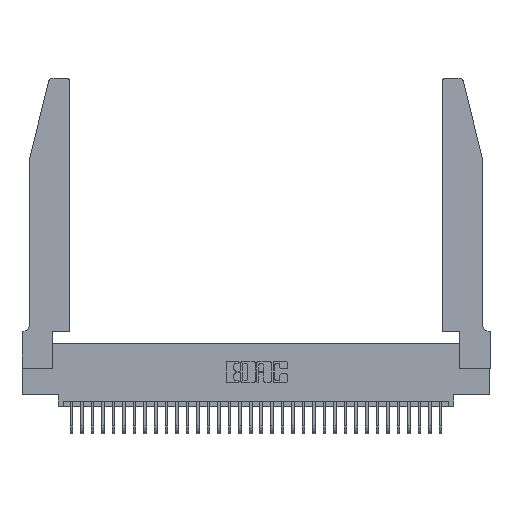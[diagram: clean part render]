
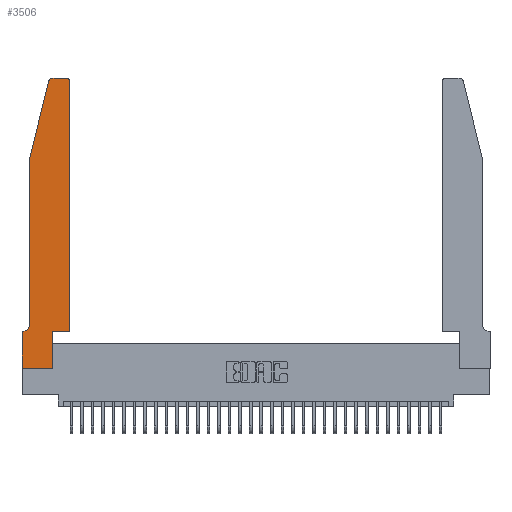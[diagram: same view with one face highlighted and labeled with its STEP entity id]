
A CAD part, top view. The second image highlights one B-rep face of the part: STEP entity #3506.
In plain terms, the highlighted planar face has unit normal (0, 0, 1).
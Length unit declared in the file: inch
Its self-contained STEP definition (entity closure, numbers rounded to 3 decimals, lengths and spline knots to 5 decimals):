
#100 = EDGE_CURVE ( 'NONE', #10285, #5975, #26874, .T. ) ;
#257 = VECTOR ( 'NONE', #12588, 39.37008 ) ;
#809 = AXIS2_PLACEMENT_3D ( 'NONE', #14384, #32097, #16927 ) ;
#1375 = VERTEX_POINT ( 'NONE', #4987 ) ;
#1424 = ORIENTED_EDGE ( 'NONE', *, *, #3995, .T. ) ;
#1667 = LINE ( 'NONE', #10837, #7676 ) ;
#1748 = ORIENTED_EDGE ( 'NONE', *, *, #4830, .T. ) ;
#1762 = DIRECTION ( 'NONE',  ( 0., 0., 1. ) ) ;
#2508 = VERTEX_POINT ( 'NONE', #12590 ) ;
#2565 = VECTOR ( 'NONE', #19138, 39.37008 ) ;
#2974 = EDGE_CURVE ( 'NONE', #5975, #3243, #23541, .T. ) ;
#3184 = CARTESIAN_POINT ( 'NONE',  ( 0.2865, 0.35, 0.37 ) ) ;
#3243 = VERTEX_POINT ( 'NONE', #20461 ) ;
#3506 = ADVANCED_FACE ( 'NONE', ( #21100 ), #26480, .T. ) ;
#3995 = EDGE_CURVE ( 'NONE', #10096, #30530, #20252, .T. ) ;
#4830 = EDGE_CURVE ( 'NONE', #26191, #29279, #29350, .T. ) ;
#4987 = CARTESIAN_POINT ( 'NONE',  ( 0.0055, 0.35, 0.37 ) ) ;
#5156 = CARTESIAN_POINT ( 'NONE',  ( 0., 0., 0.37 ) ) ;
#5867 = VECTOR ( 'NONE', #12984, 39.37008 ) ;
#5939 = VECTOR ( 'NONE', #24804, 39.37008 ) ;
#5963 = VECTOR ( 'NONE', #23634, 39.37008 ) ;
#5975 = VERTEX_POINT ( 'NONE', #12369 ) ;
#6081 = EDGE_CURVE ( 'NONE', #3243, #10096, #18925, .T. ) ;
#7092 = CARTESIAN_POINT ( 'NONE',  ( 0.0755, 2., 0.37 ) ) ;
#7093 = LINE ( 'NONE', #7507, #257 ) ;
#7507 = CARTESIAN_POINT ( 'NONE',  ( 0.4505, 0.35, 0.37 ) ) ;
#7676 = VECTOR ( 'NONE', #25961, 39.37008 ) ;
#7821 = ORIENTED_EDGE ( 'NONE', *, *, #100, .T. ) ;
#7917 = ORIENTED_EDGE ( 'NONE', *, *, #28619, .T. ) ;
#8283 = ORIENTED_EDGE ( 'NONE', *, *, #28003, .T. ) ;
#8808 = CIRCLE ( 'NONE', #809, 0.07 ) ;
#9405 = LINE ( 'NONE', #24055, #2565 ) ;
#9888 = DIRECTION ( 'NONE',  ( 0., -1., 0. ) ) ;
#10096 = VERTEX_POINT ( 'NONE', #30435 ) ;
#10285 = VERTEX_POINT ( 'NONE', #26589 ) ;
#10837 = CARTESIAN_POINT ( 'NONE',  ( 0., 0., 0.37 ) ) ;
#11023 = CARTESIAN_POINT ( 'NONE',  ( 0., 0., 0.37 ) ) ;
#11328 = CARTESIAN_POINT ( 'NONE',  ( 0., 0.35, 0.37 ) ) ;
#11965 = CARTESIAN_POINT ( 'NONE',  ( 0.25487, 2.72718, 0.37 ) ) ;
#12243 = EDGE_CURVE ( 'NONE', #1375, #18558, #29866, .T. ) ;
#12369 = CARTESIAN_POINT ( 'NONE',  ( 0.4505, 2.72, 0.37 ) ) ;
#12539 = EDGE_CURVE ( 'NONE', #30699, #2508, #1667, .T. ) ;
#12588 = DIRECTION ( 'NONE',  ( 1., 0., 0. ) ) ;
#12590 = CARTESIAN_POINT ( 'NONE',  ( 0.2865, 0., 0.37 ) ) ;
#12671 = LINE ( 'NONE', #7092, #5939 ) ;
#12984 = DIRECTION ( 'NONE',  ( 0., 1., 0. ) ) ;
#13039 = DIRECTION ( 'NONE',  ( 0., 0., 1. ) ) ;
#13126 = AXIS2_PLACEMENT_3D ( 'NONE', #11328, #13847, #31569 ) ;
#13847 = DIRECTION ( 'NONE',  ( 0., 0., 1. ) ) ;
#14384 = CARTESIAN_POINT ( 'NONE',  ( 0.0055, 0.42, 0.37 ) ) ;
#15065 = VECTOR ( 'NONE', #9888, 39.37008 ) ;
#15215 = DIRECTION ( 'NONE',  ( -1., 0., 0. ) ) ;
#15487 = EDGE_LOOP ( 'NONE', ( #26988, #1424, #8283, #1748, #27468, #16685, #23437, #31357, #21191, #7917, #7821, #29289 ) ) ;
#16685 = ORIENTED_EDGE ( 'NONE', *, *, #12243, .T. ) ;
#16927 = DIRECTION ( 'NONE',  ( -1., 0., 0. ) ) ;
#16969 = CARTESIAN_POINT ( 'NONE',  ( 0.4205, 2.72, 0.37 ) ) ;
#17240 = DIRECTION ( 'NONE',  ( -1., 0., 0. ) ) ;
#17566 = AXIS2_PLACEMENT_3D ( 'NONE', #28218, #13039, #30749 ) ;
#17757 = AXIS2_PLACEMENT_3D ( 'NONE', #16969, #1762, #19514 ) ;
#18558 = VERTEX_POINT ( 'NONE', #31623 ) ;
#18605 = LINE ( 'NONE', #11023, #5963 ) ;
#18925 = LINE ( 'NONE', #30380, #31633 ) ;
#19138 = DIRECTION ( 'NONE',  ( 0., 1., 0. ) ) ;
#19514 = DIRECTION ( 'NONE',  ( 1., 0., 0. ) ) ;
#19920 = EDGE_CURVE ( 'NONE', #29279, #1375, #8808, .T. ) ;
#20252 = CIRCLE ( 'NONE', #17566, 0.03 ) ;
#20461 = CARTESIAN_POINT ( 'NONE',  ( 0.4205, 2.75, 0.37 ) ) ;
#21100 = FACE_OUTER_BOUND ( 'NONE', #15487, .T. ) ;
#21191 = ORIENTED_EDGE ( 'NONE', *, *, #29896, .T. ) ;
#22498 = CARTESIAN_POINT ( 'NONE',  ( 0.0755, 2., 0.37 ) ) ;
#23126 = VECTOR ( 'NONE', #17240, 39.37008 ) ;
#23437 = ORIENTED_EDGE ( 'NONE', *, *, #23928, .T. ) ;
#23541 = CIRCLE ( 'NONE', #17757, 0.03 ) ;
#23634 = DIRECTION ( 'NONE',  ( 0., -1., 0. ) ) ;
#23928 = EDGE_CURVE ( 'NONE', #18558, #30699, #18605, .T. ) ;
#24055 = CARTESIAN_POINT ( 'NONE',  ( 0.2865, 0.35, 0.37 ) ) ;
#24804 = DIRECTION ( 'NONE',  ( -0.239, -0.971, 0. ) ) ;
#25481 = CARTESIAN_POINT ( 'NONE',  ( 0.4505, 0.35, 0.37 ) ) ;
#25491 = CARTESIAN_POINT ( 'NONE',  ( 0.0755, 2., 0.37 ) ) ;
#25961 = DIRECTION ( 'NONE',  ( 1., 0., 0. ) ) ;
#26191 = VERTEX_POINT ( 'NONE', #25491 ) ;
#26480 = PLANE ( 'NONE',  #13126 ) ;
#26589 = CARTESIAN_POINT ( 'NONE',  ( 0.4505, 0.35, 0.37 ) ) ;
#26874 = LINE ( 'NONE', #25481, #5867 ) ;
#26988 = ORIENTED_EDGE ( 'NONE', *, *, #6081, .T. ) ;
#27342 = CARTESIAN_POINT ( 'NONE',  ( 0.0755, 0.35, 0.37 ) ) ;
#27468 = ORIENTED_EDGE ( 'NONE', *, *, #19920, .T. ) ;
#28003 = EDGE_CURVE ( 'NONE', #30530, #26191, #12671, .T. ) ;
#28218 = CARTESIAN_POINT ( 'NONE',  ( 0.284, 2.72, 0.37 ) ) ;
#28619 = EDGE_CURVE ( 'NONE', #29496, #10285, #7093, .T. ) ;
#29279 = VERTEX_POINT ( 'NONE', #32672 ) ;
#29289 = ORIENTED_EDGE ( 'NONE', *, *, #2974, .T. ) ;
#29350 = LINE ( 'NONE', #22498, #15065 ) ;
#29496 = VERTEX_POINT ( 'NONE', #3184 ) ;
#29866 = LINE ( 'NONE', #27342, #23126 ) ;
#29896 = EDGE_CURVE ( 'NONE', #2508, #29496, #9405, .T. ) ;
#30380 = CARTESIAN_POINT ( 'NONE',  ( 0.2605, 2.75, 0.37 ) ) ;
#30435 = CARTESIAN_POINT ( 'NONE',  ( 0.284, 2.75, 0.37 ) ) ;
#30530 = VERTEX_POINT ( 'NONE', #11965 ) ;
#30699 = VERTEX_POINT ( 'NONE', #5156 ) ;
#30749 = DIRECTION ( 'NONE',  ( 1., 0., 0. ) ) ;
#31357 = ORIENTED_EDGE ( 'NONE', *, *, #12539, .T. ) ;
#31569 = DIRECTION ( 'NONE',  ( 1., 0., 0. ) ) ;
#31623 = CARTESIAN_POINT ( 'NONE',  ( 0., 0.35, 0.37 ) ) ;
#31633 = VECTOR ( 'NONE', #15215, 39.37008 ) ;
#32097 = DIRECTION ( 'NONE',  ( 0., 0., -1. ) ) ;
#32672 = CARTESIAN_POINT ( 'NONE',  ( 0.0755, 0.42, 0.37 ) ) ;
